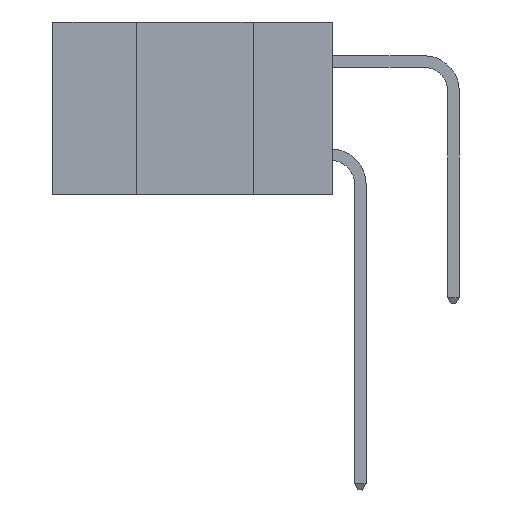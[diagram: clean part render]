
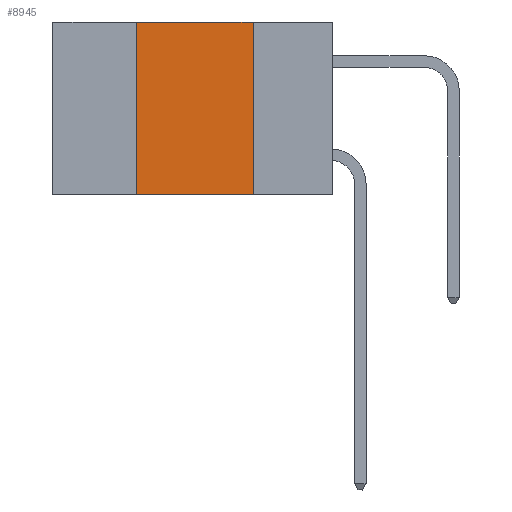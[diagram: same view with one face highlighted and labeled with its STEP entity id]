
A CAD part, left-side view. The second image highlights one B-rep face of the part: STEP entity #8945.
In plain terms, the highlighted planar face has unit normal (-1, 0, 0).
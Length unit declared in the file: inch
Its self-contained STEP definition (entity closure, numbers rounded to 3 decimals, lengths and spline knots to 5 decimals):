
#91 = EDGE_CURVE ( 'NONE', #1414, #6242, #1082, .T. ) ;
#92 = ORIENTED_EDGE ( 'NONE', *, *, #91, .F. ) ;
#297 = VERTEX_POINT ( 'NONE', #1524 ) ;
#434 = CARTESIAN_POINT ( 'NONE',  ( 0., 0.17, -0.37 ) ) ;
#654 = DIRECTION ( 'NONE',  ( 0., -1., 0. ) ) ;
#857 = VECTOR ( 'NONE', #654, 39.37008 ) ;
#1005 = LINE ( 'NONE', #7905, #4844 ) ;
#1082 = LINE ( 'NONE', #2882, #5099 ) ;
#1204 = CARTESIAN_POINT ( 'NONE',  ( 0., 0.17, 0. ) ) ;
#1414 = VERTEX_POINT ( 'NONE', #4482 ) ;
#1524 = CARTESIAN_POINT ( 'NONE',  ( 0., 0.42, -0.37 ) ) ;
#1534 = AXIS2_PLACEMENT_3D ( 'NONE', #10524, #9287, #2579 ) ;
#2217 = VERTEX_POINT ( 'NONE', #434 ) ;
#2463 = CARTESIAN_POINT ( 'NONE',  ( 0., 0.6, -0.37 ) ) ;
#2579 = DIRECTION ( 'NONE',  ( 0., 0., -1. ) ) ;
#2882 = CARTESIAN_POINT ( 'NONE',  ( 0., 0.6, 0. ) ) ;
#2976 = LINE ( 'NONE', #7829, #11598 ) ;
#3752 = ORIENTED_EDGE ( 'NONE', *, *, #5869, .T. ) ;
#4482 = CARTESIAN_POINT ( 'NONE',  ( 0., 0.42, 0. ) ) ;
#4844 = VECTOR ( 'NONE', #7844, 39.37008 ) ;
#5099 = VECTOR ( 'NONE', #8893, 39.37008 ) ;
#5869 = EDGE_CURVE ( 'NONE', #297, #2217, #11247, .T. ) ;
#6242 = VERTEX_POINT ( 'NONE', #1204 ) ;
#6748 = ORIENTED_EDGE ( 'NONE', *, *, #10129, .F. ) ;
#7769 = DIRECTION ( 'NONE',  ( 0., 0., -1. ) ) ;
#7829 = CARTESIAN_POINT ( 'NONE',  ( 0., 0.17, -0.37 ) ) ;
#7844 = DIRECTION ( 'NONE',  ( 0., 0., 1. ) ) ;
#7905 = CARTESIAN_POINT ( 'NONE',  ( 0., 0.42, -0.37 ) ) ;
#8893 = DIRECTION ( 'NONE',  ( 0., -1., 0. ) ) ;
#8945 = ADVANCED_FACE ( 'NONE', ( #10461 ), #10334, .F. ) ;
#9287 = DIRECTION ( 'NONE',  ( 1., 0., 0. ) ) ;
#10129 = EDGE_CURVE ( 'NONE', #6242, #2217, #2976, .T. ) ;
#10334 = PLANE ( 'NONE',  #1534 ) ;
#10461 = FACE_OUTER_BOUND ( 'NONE', #12015, .T. ) ;
#10488 = ORIENTED_EDGE ( 'NONE', *, *, #11064, .F. ) ;
#10524 = CARTESIAN_POINT ( 'NONE',  ( 0., 0.6, 0. ) ) ;
#11064 = EDGE_CURVE ( 'NONE', #297, #1414, #1005, .T. ) ;
#11247 = LINE ( 'NONE', #2463, #857 ) ;
#11598 = VECTOR ( 'NONE', #7769, 39.37008 ) ;
#12015 = EDGE_LOOP ( 'NONE', ( #6748, #92, #10488, #3752 ) ) ;
